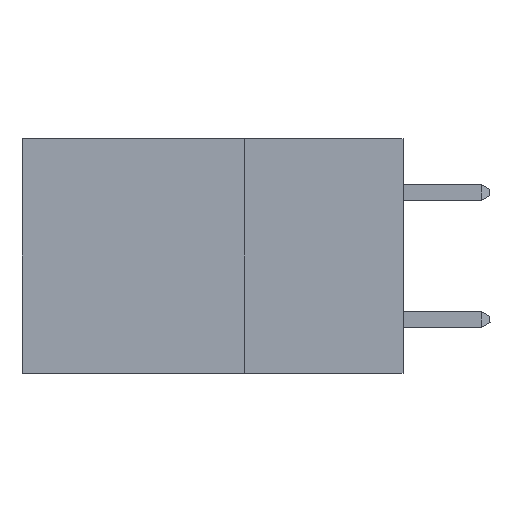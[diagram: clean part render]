
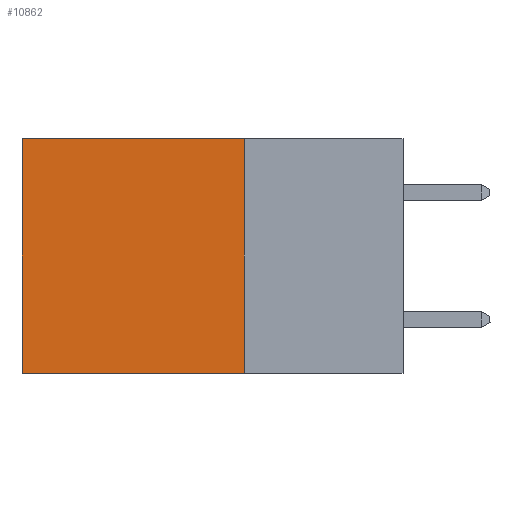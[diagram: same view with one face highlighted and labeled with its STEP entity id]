
A CAD part, left-side view. The second image highlights one B-rep face of the part: STEP entity #10862.
In plain terms, the highlighted planar face has unit normal (-1, 0, 0).
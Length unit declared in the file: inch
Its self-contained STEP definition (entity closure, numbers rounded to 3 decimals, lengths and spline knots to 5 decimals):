
#1471 = PLANE ( 'NONE',  #7300 ) ;
#3057 = VERTEX_POINT ( 'NONE', #18823 ) ;
#3804 = CARTESIAN_POINT ( 'NONE',  ( 0.2875, 0.25, 0. ) ) ;
#4741 = CARTESIAN_POINT ( 'NONE',  ( 0.2875, 0.25, 0. ) ) ;
#4939 = FACE_OUTER_BOUND ( 'NONE', #6278, .T. ) ;
#6063 = DIRECTION ( 'NONE',  ( 0., 0., -1. ) ) ;
#6278 = EDGE_LOOP ( 'NONE', ( #15408, #9233, #25245, #17205 ) ) ;
#6377 = EDGE_CURVE ( 'NONE', #11440, #10040, #18759, .T. ) ;
#7300 = AXIS2_PLACEMENT_3D ( 'NONE', #3804, #19184, #6063 ) ;
#7859 = VECTOR ( 'NONE', #27255, 39.37008 ) ;
#8037 = VECTOR ( 'NONE', #13210, 39.37008 ) ;
#9233 = ORIENTED_EDGE ( 'NONE', *, *, #6377, .F. ) ;
#9341 = EDGE_CURVE ( 'NONE', #3057, #10040, #15658, .T. ) ;
#9786 = VERTEX_POINT ( 'NONE', #23843 ) ;
#10040 = VERTEX_POINT ( 'NONE', #16044 ) ;
#10862 = ADVANCED_FACE ( 'NONE', ( #4939 ), #1471, .F. ) ;
#11069 = CARTESIAN_POINT ( 'NONE',  ( 0.2875, 0.25, 0. ) ) ;
#11440 = VERTEX_POINT ( 'NONE', #16662 ) ;
#12145 = CARTESIAN_POINT ( 'NONE',  ( 0.2875, 0.25, -0.37 ) ) ;
#12436 = VECTOR ( 'NONE', #20085, 39.37008 ) ;
#13210 = DIRECTION ( 'NONE',  ( 0., 1., 0. ) ) ;
#15408 = ORIENTED_EDGE ( 'NONE', *, *, #9341, .T. ) ;
#15658 = LINE ( 'NONE', #17217, #26500 ) ;
#16044 = CARTESIAN_POINT ( 'NONE',  ( 0.2875, 0.6, -0.37 ) ) ;
#16662 = CARTESIAN_POINT ( 'NONE',  ( 0.2875, 0.25, -0.37 ) ) ;
#17205 = ORIENTED_EDGE ( 'NONE', *, *, #17523, .T. ) ;
#17217 = CARTESIAN_POINT ( 'NONE',  ( 0.2875, 0.6, 0. ) ) ;
#17523 = EDGE_CURVE ( 'NONE', #9786, #3057, #25341, .T. ) ;
#17540 = LINE ( 'NONE', #4741, #12436 ) ;
#17632 = EDGE_CURVE ( 'NONE', #9786, #11440, #17540, .T. ) ;
#18759 = LINE ( 'NONE', #12145, #7859 ) ;
#18823 = CARTESIAN_POINT ( 'NONE',  ( 0.2875, 0.6, 0. ) ) ;
#19184 = DIRECTION ( 'NONE',  ( 1., 0., 0. ) ) ;
#19416 = DIRECTION ( 'NONE',  ( 0., 0., -1. ) ) ;
#20085 = DIRECTION ( 'NONE',  ( 0., 0., -1. ) ) ;
#23843 = CARTESIAN_POINT ( 'NONE',  ( 0.2875, 0.25, 0. ) ) ;
#25245 = ORIENTED_EDGE ( 'NONE', *, *, #17632, .F. ) ;
#25341 = LINE ( 'NONE', #11069, #8037 ) ;
#26500 = VECTOR ( 'NONE', #19416, 39.37008 ) ;
#27255 = DIRECTION ( 'NONE',  ( 0., 1., 0. ) ) ;
